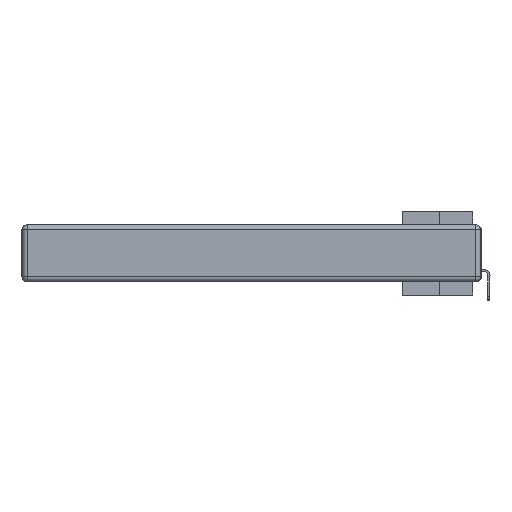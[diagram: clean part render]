
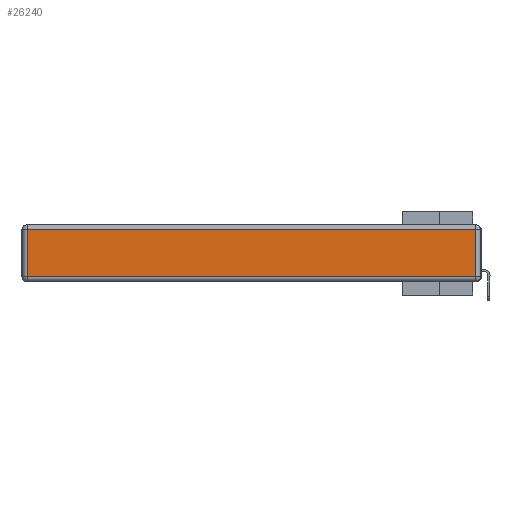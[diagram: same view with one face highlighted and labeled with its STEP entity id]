
A CAD part, left-side view. The second image highlights one B-rep face of the part: STEP entity #26240.
In plain terms, the highlighted planar face has unit normal (-1, 0, 0).
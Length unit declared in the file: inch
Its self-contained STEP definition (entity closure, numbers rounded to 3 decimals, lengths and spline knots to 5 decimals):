
#27 = VERTEX_POINT ( 'NONE', #4774 ) ;
#119 = FACE_OUTER_BOUND ( 'NONE', #29231, .T. ) ;
#801 = AXIS2_PLACEMENT_3D ( 'NONE', #13062, #30864, #10693 ) ;
#849 = CARTESIAN_POINT ( 'NONE',  ( 0., 0.03, -0.03 ) ) ;
#1149 = VECTOR ( 'NONE', #13794, 39.37008 ) ;
#2719 = PLANE ( 'NONE',  #801 ) ;
#3478 = EDGE_CURVE ( 'NONE', #7820, #5006, #27614, .T. ) ;
#4774 = CARTESIAN_POINT ( 'NONE',  ( 0., 2.72, -0.03 ) ) ;
#5006 = VERTEX_POINT ( 'NONE', #25026 ) ;
#7820 = VERTEX_POINT ( 'NONE', #8170 ) ;
#7910 = LINE ( 'NONE', #29079, #1149 ) ;
#8087 = LINE ( 'NONE', #11119, #32004 ) ;
#8157 = VERTEX_POINT ( 'NONE', #849 ) ;
#8170 = CARTESIAN_POINT ( 'NONE',  ( 0., 2.72, -0.313 ) ) ;
#8844 = VECTOR ( 'NONE', #17386, 39.37008 ) ;
#9104 = EDGE_CURVE ( 'NONE', #27, #7820, #8087, .T. ) ;
#9839 = EDGE_CURVE ( 'NONE', #5006, #8157, #19012, .T. ) ;
#10654 = DIRECTION ( 'NONE',  ( 0., 0., -1. ) ) ;
#10693 = DIRECTION ( 'NONE',  ( 0., 0., 1. ) ) ;
#11119 = CARTESIAN_POINT ( 'NONE',  ( 0., 2.72, -0.343 ) ) ;
#13062 = CARTESIAN_POINT ( 'NONE',  ( 0., 0., -0.343 ) ) ;
#13794 = DIRECTION ( 'NONE',  ( 0., 1., 0. ) ) ;
#14870 = ORIENTED_EDGE ( 'NONE', *, *, #9839, .T. ) ;
#16595 = CARTESIAN_POINT ( 'NONE',  ( 0., 0.03, -0.343 ) ) ;
#17386 = DIRECTION ( 'NONE',  ( 0., -1., 0. ) ) ;
#17416 = ORIENTED_EDGE ( 'NONE', *, *, #9104, .T. ) ;
#18047 = EDGE_CURVE ( 'NONE', #8157, #27, #7910, .T. ) ;
#19012 = LINE ( 'NONE', #16595, #25394 ) ;
#25026 = CARTESIAN_POINT ( 'NONE',  ( 0., 0.03, -0.313 ) ) ;
#25394 = VECTOR ( 'NONE', #27217, 39.37008 ) ;
#25471 = ORIENTED_EDGE ( 'NONE', *, *, #3478, .T. ) ;
#26240 = ADVANCED_FACE ( 'NONE', ( #119 ), #2719, .T. ) ;
#27217 = DIRECTION ( 'NONE',  ( 0., 0., 1. ) ) ;
#27614 = LINE ( 'NONE', #32996, #8844 ) ;
#29079 = CARTESIAN_POINT ( 'NONE',  ( 0., 2.75, -0.03 ) ) ;
#29231 = EDGE_LOOP ( 'NONE', ( #25471, #14870, #31963, #17416 ) ) ;
#30864 = DIRECTION ( 'NONE',  ( -1., 0., 0. ) ) ;
#31963 = ORIENTED_EDGE ( 'NONE', *, *, #18047, .T. ) ;
#32004 = VECTOR ( 'NONE', #10654, 39.37008 ) ;
#32996 = CARTESIAN_POINT ( 'NONE',  ( 0., 0., -0.313 ) ) ;
